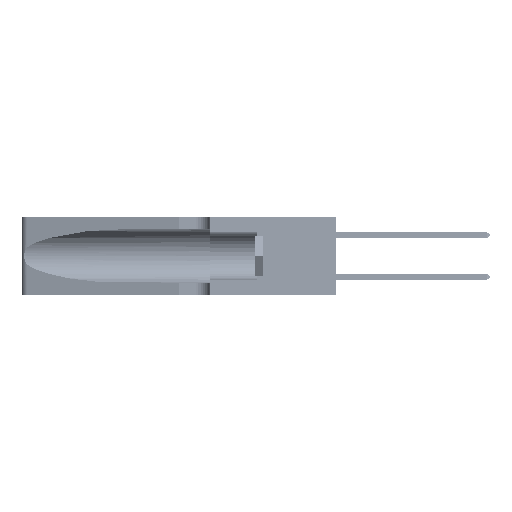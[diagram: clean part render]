
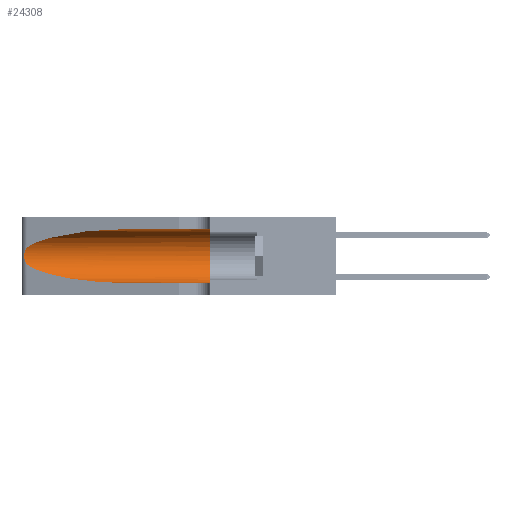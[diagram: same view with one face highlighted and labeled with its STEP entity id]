
A CAD part, left-side view. The second image highlights one B-rep face of the part: STEP entity #24308.
In plain terms, the highlighted cylindrical face has radius 3.308 mm (diameter 6.617 mm), a partial arc.
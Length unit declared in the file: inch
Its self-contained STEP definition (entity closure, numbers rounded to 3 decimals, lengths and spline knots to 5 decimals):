
#896 = VERTEX_POINT ( 'NONE', #47267 ) ;
#1346 = CARTESIAN_POINT ( 'NONE',  ( 0.25555, 1.22993, 0.14849 ) ) ;
#4316 = CIRCLE ( 'NONE', #37481, 0.13025 ) ;
#5147 = EDGE_CURVE ( 'NONE', #36196, #19774, #33838, .T. ) ;
#6152 = VECTOR ( 'NONE', #47047, 39.37008 ) ;
#7010 = CARTESIAN_POINT ( 'NONE',  ( 0.1305, 0.72297, 0.31525 ) ) ;
#8952 = VERTEX_POINT ( 'NONE', #45501 ) ;
#9051 = CARTESIAN_POINT ( 'NONE',  ( 0.1305, 0.72297, 0.05475 ) ) ;
#9053 = VECTOR ( 'NONE', #18976, 39.37008 ) ;
#9814 = CARTESIAN_POINT ( 'NONE',  ( 0.25787, 1.23484, 0.2124 ) ) ;
#10866 = DIRECTION ( 'NONE',  ( 0., -1., 0. ) ) ;
#11105 = ORIENTED_EDGE ( 'NONE', *, *, #26830, .F. ) ;
#11482 = CARTESIAN_POINT ( 'NONE',  ( 0.1305, 0.72297, 0.05475 ) ) ;
#11556 = ORIENTED_EDGE ( 'NONE', *, *, #42997, .T. ) ;
#13704 = ORIENTED_EDGE ( 'NONE', *, *, #46264, .T. ) ;
#14059 = CARTESIAN_POINT ( 'NONE',  ( 0.26018, 1.23835, 0.19895 ) ) ;
#14171 = ORIENTED_EDGE ( 'NONE', *, *, #54372, .T. ) ;
#15168 = DIRECTION ( 'NONE',  ( 0., 1., 0. ) ) ;
#15538 = CARTESIAN_POINT ( 'NONE',  ( 0.25487, 1.22718, 0.22369 ) ) ;
#16073 = AXIS2_PLACEMENT_3D ( 'NONE', #27744, #10866, #48538 ) ;
#17250 = ORIENTED_EDGE ( 'NONE', *, *, #5147, .T. ) ;
#18331 = CARTESIAN_POINT ( 'NONE',  ( 0.26075, 1.23896, 0.178 ) ) ;
#18862 = CARTESIAN_POINT ( 'NONE',  ( 0.1305, 0.35, 0.05475 ) ) ;
#18976 = DIRECTION ( 'NONE',  ( 0., -1., 0. ) ) ;
#19774 = VERTEX_POINT ( 'NONE', #9051 ) ;
#19831 = CARTESIAN_POINT ( 'NONE',  ( 0.2373, 1.15595, 0.08982 ) ) ;
#19888 = CYLINDRICAL_SURFACE ( 'NONE', #16073, 0.13025 ) ;
#22587 = CARTESIAN_POINT ( 'NONE',  ( 0.25856, 1.23593, 0.16098 ) ) ;
#24308 = ADVANCED_FACE ( 'NONE', ( #42238 ), #19888, .F. ) ;
#24395 = ORIENTED_EDGE ( 'NONE', *, *, #43152, .F. ) ;
#25724 =( BOUNDED_CURVE ( )  B_SPLINE_CURVE ( 3, ( #7010, #32382, #40783, #15538 ),
 .UNSPECIFIED., .F., .F. ) 
 B_SPLINE_CURVE_WITH_KNOTS ( ( 4, 4 ),
 ( 1.5708, 2.84003 ),
 .UNSPECIFIED. ) 
 CURVE ( )  GEOMETRIC_REPRESENTATION_ITEM ( )  RATIONAL_B_SPLINE_CURVE ( ( 1., 0.87, 0.87, 1. ) ) 
 REPRESENTATION_ITEM ( '' )  );
#26167 = VERTEX_POINT ( 'NONE', #18862 ) ;
#26403 = CARTESIAN_POINT ( 'NONE',  ( 0.1305, 0.35, 0.31525 ) ) ;
#26830 = EDGE_CURVE ( 'NONE', #896, #34776, #31592, .T. ) ;
#26846 = CARTESIAN_POINT ( 'NONE',  ( 0.25639, 1.23186, 0.15144 ) ) ;
#27314 = CARTESIAN_POINT ( 'NONE',  ( 0.1305, 1.61858, 0.31525 ) ) ;
#27744 = CARTESIAN_POINT ( 'NONE',  ( 0.1305, 1.61858, 0.185 ) ) ;
#30939 = CARTESIAN_POINT ( 'NONE',  ( 0.25487, 1.22718, 0.22369 ) ) ;
#31122 = CARTESIAN_POINT ( 'NONE',  ( 0.25487, 1.22718, 0.14631 ) ) ;
#31592 = LINE ( 'NONE', #27314, #9053 ) ;
#32382 = CARTESIAN_POINT ( 'NONE',  ( 0.18966, 0.96281, 0.31525 ) ) ;
#33838 =( BOUNDED_CURVE ( )  B_SPLINE_CURVE ( 3, ( #53351, #19831, #40794, #11482 ),
 .UNSPECIFIED., .F., .F. ) 
 B_SPLINE_CURVE_WITH_KNOTS ( ( 4, 4 ),
 ( 3.44316, 4.71239 ),
 .UNSPECIFIED. ) 
 CURVE ( )  GEOMETRIC_REPRESENTATION_ITEM ( )  RATIONAL_B_SPLINE_CURVE ( ( 1., 0.87, 0.87, 1. ) ) 
 REPRESENTATION_ITEM ( '' )  );
#34488 = CARTESIAN_POINT ( 'NONE',  ( 0.1305, 1.61858, 0.05475 ) ) ;
#34776 = VERTEX_POINT ( 'NONE', #26403 ) ;
#35133 = CARTESIAN_POINT ( 'NONE',  ( 0.25639, 1.23184, 0.21858 ) ) ;
#36196 = VERTEX_POINT ( 'NONE', #40380 ) ;
#37481 = AXIS2_PLACEMENT_3D ( 'NONE', #40385, #15168, #44585 ) ;
#39324 = CARTESIAN_POINT ( 'NONE',  ( 0.25854, 1.2359, 0.20912 ) ) ;
#40380 = CARTESIAN_POINT ( 'NONE',  ( 0.25487, 1.22718, 0.14631 ) ) ;
#40385 = CARTESIAN_POINT ( 'NONE',  ( 0.1305, 0.35, 0.185 ) ) ;
#40783 = CARTESIAN_POINT ( 'NONE',  ( 0.2373, 1.15595, 0.28018 ) ) ;
#40794 = CARTESIAN_POINT ( 'NONE',  ( 0.18966, 0.96281, 0.05475 ) ) ;
#42238 = FACE_OUTER_BOUND ( 'NONE', #52466, .T. ) ;
#42997 = EDGE_CURVE ( 'NONE', #8952, #36196, #45187, .T. ) ;
#43152 = EDGE_CURVE ( 'NONE', #34776, #26167, #4316, .T. ) ;
#43508 = CARTESIAN_POINT ( 'NONE',  ( 0.26075, 1.23896, 0.19203 ) ) ;
#44585 = DIRECTION ( 'NONE',  ( 0., 0., 1. ) ) ;
#45187 = B_SPLINE_CURVE_WITH_KNOTS ( 'NONE', 3,
 ( #30939, #51696, #35133, #9814, #39324, #14059, #43508, #18331, #47685, #22587, #51862, #26846, #1346, #31122 ),
 .UNSPECIFIED., .F., .F.,
 ( 4, 2, 2, 2, 2, 2, 4 ),
 ( 0., 0.00027, 0.00053, 0.00107, 0.0016, 0.00187, 0.00214 ),
 .UNSPECIFIED. ) ;
#45501 = CARTESIAN_POINT ( 'NONE',  ( 0.25487, 1.22718, 0.22369 ) ) ;
#46264 = EDGE_CURVE ( 'NONE', #896, #8952, #25724, .T. ) ;
#47047 = DIRECTION ( 'NONE',  ( 0., -1., 0. ) ) ;
#47267 = CARTESIAN_POINT ( 'NONE',  ( 0.1305, 0.72297, 0.31525 ) ) ;
#47685 = CARTESIAN_POINT ( 'NONE',  ( 0.26017, 1.23833, 0.17102 ) ) ;
#48538 = DIRECTION ( 'NONE',  ( 0., 0., -1. ) ) ;
#49610 = LINE ( 'NONE', #34488, #6152 ) ;
#51696 = CARTESIAN_POINT ( 'NONE',  ( 0.25555, 1.22994, 0.2215 ) ) ;
#51862 = CARTESIAN_POINT ( 'NONE',  ( 0.25789, 1.23486, 0.15765 ) ) ;
#52466 = EDGE_LOOP ( 'NONE', ( #13704, #11556, #17250, #14171, #24395, #11105 ) ) ;
#53351 = CARTESIAN_POINT ( 'NONE',  ( 0.25487, 1.22718, 0.14631 ) ) ;
#54372 = EDGE_CURVE ( 'NONE', #19774, #26167, #49610, .T. ) ;
